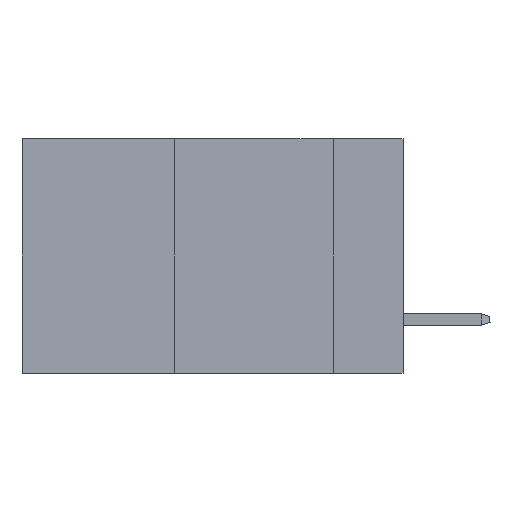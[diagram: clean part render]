
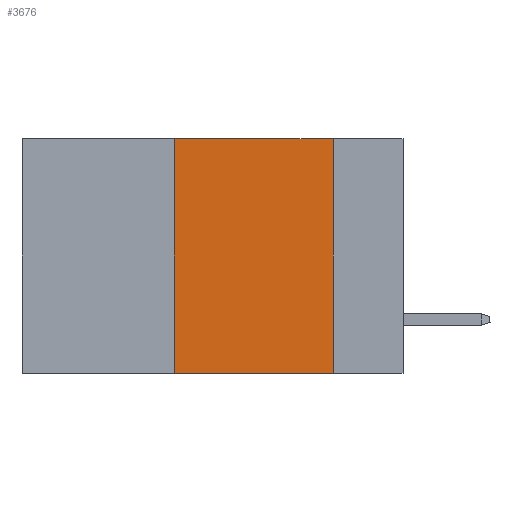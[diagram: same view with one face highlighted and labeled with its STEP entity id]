
A CAD part, left-side view. The second image highlights one B-rep face of the part: STEP entity #3676.
In plain terms, the highlighted planar face has unit normal (-1, 0, 0).
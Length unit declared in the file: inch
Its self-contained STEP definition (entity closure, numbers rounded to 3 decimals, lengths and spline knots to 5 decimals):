
#221 = DIRECTION ( 'NONE',  ( 0., -1., 0. ) ) ;
#1470 = AXIS2_PLACEMENT_3D ( 'NONE', #42543, #27084, #38162 ) ;
#3676 = ADVANCED_FACE ( 'NONE', ( #22958 ), #26313, .F. ) ;
#3785 = EDGE_CURVE ( 'NONE', #20923, #5764, #34554, .T. ) ;
#5764 = VERTEX_POINT ( 'NONE', #18745 ) ;
#7409 = EDGE_LOOP ( 'NONE', ( #29913, #45947, #42046, #8094 ) ) ;
#8094 = ORIENTED_EDGE ( 'NONE', *, *, #12222, .T. ) ;
#8140 = CARTESIAN_POINT ( 'NONE',  ( 0., 0.11, 0. ) ) ;
#10792 = VECTOR ( 'NONE', #221, 39.37008 ) ;
#11515 = CARTESIAN_POINT ( 'NONE',  ( 0., 0.36, 0. ) ) ;
#12102 = LINE ( 'NONE', #50477, #10792 ) ;
#12222 = EDGE_CURVE ( 'NONE', #46900, #35674, #12102, .T. ) ;
#12342 = VECTOR ( 'NONE', #14952, 39.37008 ) ;
#14952 = DIRECTION ( 'NONE',  ( 0., 0., 1. ) ) ;
#14983 = DIRECTION ( 'NONE',  ( 0., -1., 0. ) ) ;
#15496 = VECTOR ( 'NONE', #14983, 39.37008 ) ;
#18745 = CARTESIAN_POINT ( 'NONE',  ( 0., 0.11, 0. ) ) ;
#20923 = VERTEX_POINT ( 'NONE', #11515 ) ;
#22110 = VECTOR ( 'NONE', #27429, 39.37008 ) ;
#22958 = FACE_OUTER_BOUND ( 'NONE', #7409, .T. ) ;
#26313 = PLANE ( 'NONE',  #1470 ) ;
#27084 = DIRECTION ( 'NONE',  ( 1., 0., 0. ) ) ;
#27429 = DIRECTION ( 'NONE',  ( 0., 0., -1. ) ) ;
#29913 = ORIENTED_EDGE ( 'NONE', *, *, #39201, .F. ) ;
#34520 = CARTESIAN_POINT ( 'NONE',  ( 0., 0.36, 0. ) ) ;
#34554 = LINE ( 'NONE', #50275, #15496 ) ;
#35674 = VERTEX_POINT ( 'NONE', #45289 ) ;
#38162 = DIRECTION ( 'NONE',  ( 0., 0., -1. ) ) ;
#39201 = EDGE_CURVE ( 'NONE', #5764, #35674, #43150, .T. ) ;
#40313 = EDGE_CURVE ( 'NONE', #46900, #20923, #46116, .T. ) ;
#42046 = ORIENTED_EDGE ( 'NONE', *, *, #40313, .F. ) ;
#42543 = CARTESIAN_POINT ( 'NONE',  ( 0., 0.6, 0. ) ) ;
#43150 = LINE ( 'NONE', #8140, #22110 ) ;
#45289 = CARTESIAN_POINT ( 'NONE',  ( 0., 0.11, -0.37 ) ) ;
#45947 = ORIENTED_EDGE ( 'NONE', *, *, #3785, .F. ) ;
#46116 = LINE ( 'NONE', #34520, #12342 ) ;
#46900 = VERTEX_POINT ( 'NONE', #49049 ) ;
#49049 = CARTESIAN_POINT ( 'NONE',  ( 0., 0.36, -0.37 ) ) ;
#50275 = CARTESIAN_POINT ( 'NONE',  ( 0., 0.6, 0. ) ) ;
#50477 = CARTESIAN_POINT ( 'NONE',  ( 0., 0.6, -0.37 ) ) ;
